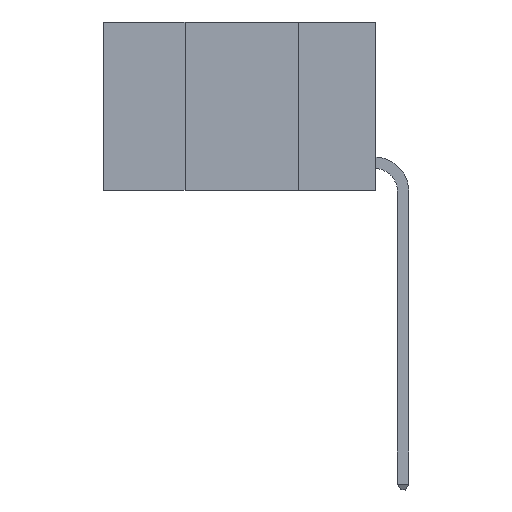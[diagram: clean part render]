
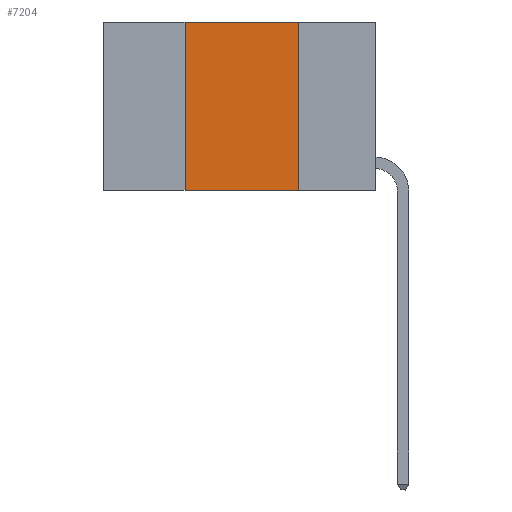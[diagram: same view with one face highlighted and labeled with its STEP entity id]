
A CAD part, left-side view. The second image highlights one B-rep face of the part: STEP entity #7204.
In plain terms, the highlighted planar face has unit normal (-1, 0, 0).
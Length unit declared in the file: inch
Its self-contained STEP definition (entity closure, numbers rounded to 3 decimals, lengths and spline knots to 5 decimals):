
#15 = DIRECTION ( 'NONE',  ( 0., 0., -1. ) ) ;
#942 = ORIENTED_EDGE ( 'NONE', *, *, #10151, .F. ) ;
#1273 = ORIENTED_EDGE ( 'NONE', *, *, #11119, .F. ) ;
#2324 = EDGE_LOOP ( 'NONE', ( #942, #9166, #1273, #6825 ) ) ;
#2604 = CARTESIAN_POINT ( 'NONE',  ( 0., 0.17, -0.37 ) ) ;
#2765 = VERTEX_POINT ( 'NONE', #2604 ) ;
#2893 = EDGE_CURVE ( 'NONE', #11890, #3131, #5809, .T. ) ;
#2949 = DIRECTION ( 'NONE',  ( 0., 0., -1. ) ) ;
#3092 = CARTESIAN_POINT ( 'NONE',  ( 0., 0.42, 0. ) ) ;
#3131 = VERTEX_POINT ( 'NONE', #6816 ) ;
#3321 = DIRECTION ( 'NONE',  ( 0., 0., 1. ) ) ;
#3633 = VECTOR ( 'NONE', #11173, 39.37008 ) ;
#3724 = AXIS2_PLACEMENT_3D ( 'NONE', #12244, #6333, #15 ) ;
#3954 = CARTESIAN_POINT ( 'NONE',  ( 0., 0.42, -0.37 ) ) ;
#5295 = PLANE ( 'NONE',  #3724 ) ;
#5450 = VECTOR ( 'NONE', #3321, 39.37008 ) ;
#5476 = VECTOR ( 'NONE', #2949, 39.37008 ) ;
#5480 = VECTOR ( 'NONE', #10468, 39.37008 ) ;
#5809 = LINE ( 'NONE', #6518, #5480 ) ;
#6094 = LINE ( 'NONE', #10409, #5450 ) ;
#6333 = DIRECTION ( 'NONE',  ( 1., 0., 0. ) ) ;
#6518 = CARTESIAN_POINT ( 'NONE',  ( 0., 0.6, 0. ) ) ;
#6816 = CARTESIAN_POINT ( 'NONE',  ( 0., 0.17, 0. ) ) ;
#6825 = ORIENTED_EDGE ( 'NONE', *, *, #11560, .T. ) ;
#7204 = ADVANCED_FACE ( 'NONE', ( #10022 ), #5295, .F. ) ;
#7704 = VERTEX_POINT ( 'NONE', #3954 ) ;
#8454 = LINE ( 'NONE', #10036, #5476 ) ;
#9166 = ORIENTED_EDGE ( 'NONE', *, *, #2893, .F. ) ;
#9358 = LINE ( 'NONE', #12138, #3633 ) ;
#10022 = FACE_OUTER_BOUND ( 'NONE', #2324, .T. ) ;
#10036 = CARTESIAN_POINT ( 'NONE',  ( 0., 0.17, 0. ) ) ;
#10151 = EDGE_CURVE ( 'NONE', #3131, #2765, #8454, .T. ) ;
#10409 = CARTESIAN_POINT ( 'NONE',  ( 0., 0.42, 0. ) ) ;
#10468 = DIRECTION ( 'NONE',  ( 0., -1., 0. ) ) ;
#11119 = EDGE_CURVE ( 'NONE', #7704, #11890, #6094, .T. ) ;
#11173 = DIRECTION ( 'NONE',  ( 0., -1., 0. ) ) ;
#11560 = EDGE_CURVE ( 'NONE', #7704, #2765, #9358, .T. ) ;
#11890 = VERTEX_POINT ( 'NONE', #3092 ) ;
#12138 = CARTESIAN_POINT ( 'NONE',  ( 0., 0.6, -0.37 ) ) ;
#12244 = CARTESIAN_POINT ( 'NONE',  ( 0., 0.6, 0. ) ) ;
